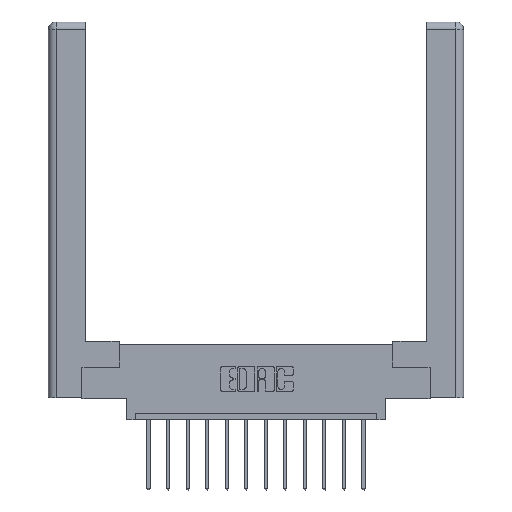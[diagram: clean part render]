
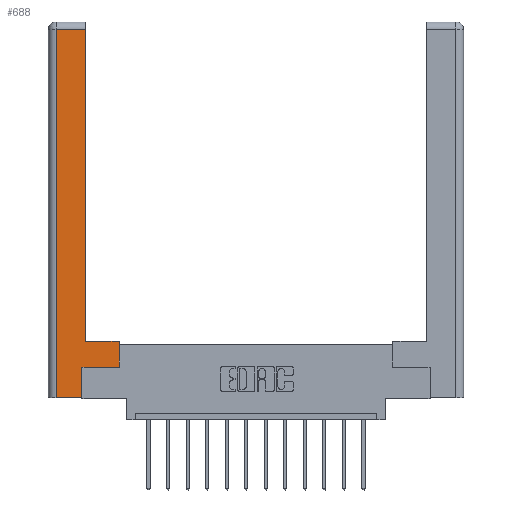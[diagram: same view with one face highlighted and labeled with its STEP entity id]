
A CAD part, top view. The second image highlights one B-rep face of the part: STEP entity #688.
In plain terms, the highlighted planar face has unit normal (0, 0, 1).
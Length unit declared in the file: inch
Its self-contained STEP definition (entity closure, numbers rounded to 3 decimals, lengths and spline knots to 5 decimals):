
#538 = DIRECTION ( 'NONE',  ( 0., 0., -1. ) ) ;
#549 = ORIENTED_EDGE ( 'NONE', *, *, #1926, .T. ) ;
#688 = ADVANCED_FACE ( 'NONE', ( #5141 ), #12553, .F. ) ;
#854 = LINE ( 'NONE', #13836, #6122 ) ;
#921 = VERTEX_POINT ( 'NONE', #3751 ) ;
#1053 = VECTOR ( 'NONE', #3222, 39.37008 ) ;
#1221 = VERTEX_POINT ( 'NONE', #8408 ) ;
#1285 = ORIENTED_EDGE ( 'NONE', *, *, #7875, .T. ) ;
#1366 = VECTOR ( 'NONE', #9229, 39.37008 ) ;
#1700 = DIRECTION ( 'NONE',  ( 0., 1., 0. ) ) ;
#1885 = LINE ( 'NONE', #6136, #14344 ) ;
#1926 = EDGE_CURVE ( 'NONE', #11825, #8290, #9449, .T. ) ;
#2131 = CARTESIAN_POINT ( 'NONE',  ( 0.265, 0., 0. ) ) ;
#2632 = VECTOR ( 'NONE', #4613, 39.37008 ) ;
#2645 = LINE ( 'NONE', #5159, #14339 ) ;
#2787 = LINE ( 'NONE', #13564, #3510 ) ;
#3153 = CARTESIAN_POINT ( 'NONE',  ( 0.0615, 2.94, 0. ) ) ;
#3222 = DIRECTION ( 'NONE',  ( -1., 0., 0. ) ) ;
#3223 = EDGE_CURVE ( 'NONE', #11338, #1221, #5828, .T. ) ;
#3510 = VECTOR ( 'NONE', #12407, 39.37008 ) ;
#3751 = CARTESIAN_POINT ( 'NONE',  ( 0.0615, 0., 0. ) ) ;
#3878 = DIRECTION ( 'NONE',  ( 1., 0., 0. ) ) ;
#4130 = AXIS2_PLACEMENT_3D ( 'NONE', #10080, #538, #12499 ) ;
#4613 = DIRECTION ( 'NONE',  ( 0., 1., 0. ) ) ;
#4825 = EDGE_CURVE ( 'NONE', #8955, #11338, #15208, .T. ) ;
#5141 = FACE_OUTER_BOUND ( 'NONE', #8481, .T. ) ;
#5159 = CARTESIAN_POINT ( 'NONE',  ( 0.565, 0.245, 0. ) ) ;
#5828 = LINE ( 'NONE', #13132, #2632 ) ;
#6122 = VECTOR ( 'NONE', #1700, 39.37008 ) ;
#6136 = CARTESIAN_POINT ( 'NONE',  ( 0.0615, 0., 0. ) ) ;
#6373 = DIRECTION ( 'NONE',  ( 1., 0., 0. ) ) ;
#6827 = VERTEX_POINT ( 'NONE', #13852 ) ;
#7366 = ORIENTED_EDGE ( 'NONE', *, *, #15041, .T. ) ;
#7523 = VECTOR ( 'NONE', #6373, 39.37008 ) ;
#7541 = CARTESIAN_POINT ( 'NONE',  ( 0.265, 0., 0. ) ) ;
#7875 = EDGE_CURVE ( 'NONE', #14261, #921, #1885, .T. ) ;
#8290 = VERTEX_POINT ( 'NONE', #8895 ) ;
#8408 = CARTESIAN_POINT ( 'NONE',  ( 0.295, 2.94, 0. ) ) ;
#8481 = EDGE_LOOP ( 'NONE', ( #9493, #7366, #1285, #8796, #549, #14025, #8612, #13674 ) ) ;
#8612 = ORIENTED_EDGE ( 'NONE', *, *, #11345, .T. ) ;
#8796 = ORIENTED_EDGE ( 'NONE', *, *, #14449, .T. ) ;
#8895 = CARTESIAN_POINT ( 'NONE',  ( 0.265, 0.245, 0. ) ) ;
#8955 = VERTEX_POINT ( 'NONE', #14265 ) ;
#9229 = DIRECTION ( 'NONE',  ( 0., 1., 0. ) ) ;
#9275 = CARTESIAN_POINT ( 'NONE',  ( 0.265, 0.245, 0. ) ) ;
#9315 = CARTESIAN_POINT ( 'NONE',  ( 0.295, 0.45, 0. ) ) ;
#9449 = LINE ( 'NONE', #9275, #1366 ) ;
#9493 = ORIENTED_EDGE ( 'NONE', *, *, #3223, .T. ) ;
#10080 = CARTESIAN_POINT ( 'NONE',  ( 0., 0., 0. ) ) ;
#10197 = CARTESIAN_POINT ( 'NONE',  ( 0.295, 0.45, 0. ) ) ;
#11338 = VERTEX_POINT ( 'NONE', #10197 ) ;
#11345 = EDGE_CURVE ( 'NONE', #6827, #8955, #854, .T. ) ;
#11825 = VERTEX_POINT ( 'NONE', #2131 ) ;
#12029 = LINE ( 'NONE', #7541, #7523 ) ;
#12407 = DIRECTION ( 'NONE',  ( -1., 0., 0. ) ) ;
#12499 = DIRECTION ( 'NONE',  ( -1., 0., 0. ) ) ;
#12553 = PLANE ( 'NONE',  #4130 ) ;
#12799 = EDGE_CURVE ( 'NONE', #8290, #6827, #2645, .T. ) ;
#13132 = CARTESIAN_POINT ( 'NONE',  ( 0.295, 3., 0. ) ) ;
#13564 = CARTESIAN_POINT ( 'NONE',  ( 0.0615, 2.94, 0. ) ) ;
#13674 = ORIENTED_EDGE ( 'NONE', *, *, #4825, .T. ) ;
#13836 = CARTESIAN_POINT ( 'NONE',  ( 0.565, 0.45, 0. ) ) ;
#13852 = CARTESIAN_POINT ( 'NONE',  ( 0.565, 0.245, 0. ) ) ;
#14025 = ORIENTED_EDGE ( 'NONE', *, *, #12799, .T. ) ;
#14261 = VERTEX_POINT ( 'NONE', #3153 ) ;
#14265 = CARTESIAN_POINT ( 'NONE',  ( 0.565, 0.45, 0. ) ) ;
#14339 = VECTOR ( 'NONE', #3878, 39.37008 ) ;
#14344 = VECTOR ( 'NONE', #14579, 39.37008 ) ;
#14449 = EDGE_CURVE ( 'NONE', #921, #11825, #12029, .T. ) ;
#14579 = DIRECTION ( 'NONE',  ( 0., -1., 0. ) ) ;
#15041 = EDGE_CURVE ( 'NONE', #1221, #14261, #2787, .T. ) ;
#15208 = LINE ( 'NONE', #9315, #1053 ) ;
